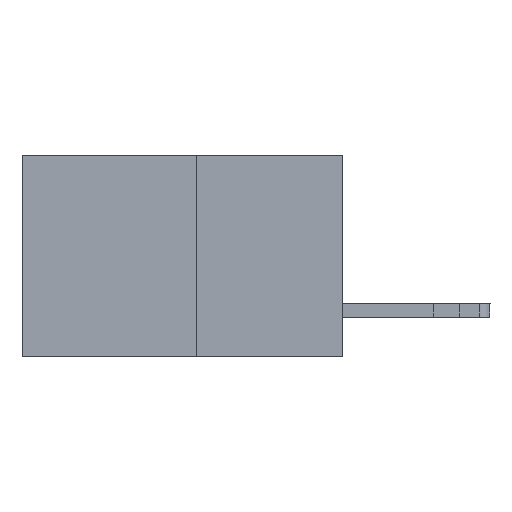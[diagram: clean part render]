
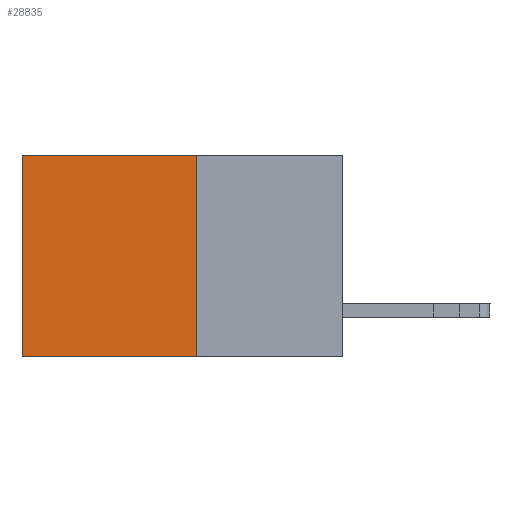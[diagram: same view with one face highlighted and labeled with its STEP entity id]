
A CAD part, left-side view. The second image highlights one B-rep face of the part: STEP entity #28835.
In plain terms, the highlighted planar face has unit normal (-1, 0, 0).
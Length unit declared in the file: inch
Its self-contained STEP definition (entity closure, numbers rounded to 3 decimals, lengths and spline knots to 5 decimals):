
#1120 = EDGE_CURVE ( 'NONE', #22946, #15707, #29380, .T. ) ;
#2297 = VECTOR ( 'NONE', #22129, 39.37008 ) ;
#2788 = ORIENTED_EDGE ( 'NONE', *, *, #28960, .T. ) ;
#3048 = VECTOR ( 'NONE', #19671, 39.37008 ) ;
#3437 = VECTOR ( 'NONE', #21261, 39.37008 ) ;
#4026 = CARTESIAN_POINT ( 'NONE',  ( 0.277, 0.27, -0.37 ) ) ;
#4163 = DIRECTION ( 'NONE',  ( 0., 0., -1. ) ) ;
#6447 = FACE_OUTER_BOUND ( 'NONE', #23843, .T. ) ;
#8493 = ORIENTED_EDGE ( 'NONE', *, *, #1120, .F. ) ;
#11939 = ORIENTED_EDGE ( 'NONE', *, *, #29833, .T. ) ;
#14759 = CARTESIAN_POINT ( 'NONE',  ( 0.277, 0.59, -0.37 ) ) ;
#15707 = VERTEX_POINT ( 'NONE', #4026 ) ;
#16087 = PLANE ( 'NONE',  #25139 ) ;
#17292 = CARTESIAN_POINT ( 'NONE',  ( 0.277, 0.27, -0.37 ) ) ;
#18547 = DIRECTION ( 'NONE',  ( 1., 0., 0. ) ) ;
#19671 = DIRECTION ( 'NONE',  ( 0., 0., -1. ) ) ;
#20452 = VERTEX_POINT ( 'NONE', #29976 ) ;
#20935 = VERTEX_POINT ( 'NONE', #29733 ) ;
#21261 = DIRECTION ( 'NONE',  ( 0., 1., 0. ) ) ;
#21481 = LINE ( 'NONE', #17292, #2297 ) ;
#22129 = DIRECTION ( 'NONE',  ( 0., 1., 0. ) ) ;
#22219 = LINE ( 'NONE', #14759, #3048 ) ;
#22622 = LINE ( 'NONE', #30965, #3437 ) ;
#22835 = DIRECTION ( 'NONE',  ( 0., 0., -1. ) ) ;
#22946 = VERTEX_POINT ( 'NONE', #30855 ) ;
#23843 = EDGE_LOOP ( 'NONE', ( #11939, #27231, #8493, #2788 ) ) ;
#25139 = AXIS2_PLACEMENT_3D ( 'NONE', #30658, #18547, #4163 ) ;
#25843 = EDGE_CURVE ( 'NONE', #15707, #20935, #21481, .T. ) ;
#27231 = ORIENTED_EDGE ( 'NONE', *, *, #25843, .F. ) ;
#28835 = ADVANCED_FACE ( 'NONE', ( #6447 ), #16087, .F. ) ;
#28942 = CARTESIAN_POINT ( 'NONE',  ( 0.277, 0.27, -0.37 ) ) ;
#28960 = EDGE_CURVE ( 'NONE', #22946, #20452, #22622, .T. ) ;
#29380 = LINE ( 'NONE', #28942, #30145 ) ;
#29733 = CARTESIAN_POINT ( 'NONE',  ( 0.277, 0.59, -0.37 ) ) ;
#29833 = EDGE_CURVE ( 'NONE', #20452, #20935, #22219, .T. ) ;
#29976 = CARTESIAN_POINT ( 'NONE',  ( 0.277, 0.59, 0. ) ) ;
#30145 = VECTOR ( 'NONE', #22835, 39.37008 ) ;
#30658 = CARTESIAN_POINT ( 'NONE',  ( 0.277, 0.27, -0.37 ) ) ;
#30855 = CARTESIAN_POINT ( 'NONE',  ( 0.277, 0.27, 0. ) ) ;
#30965 = CARTESIAN_POINT ( 'NONE',  ( 0.277, 0.27, 0. ) ) ;
